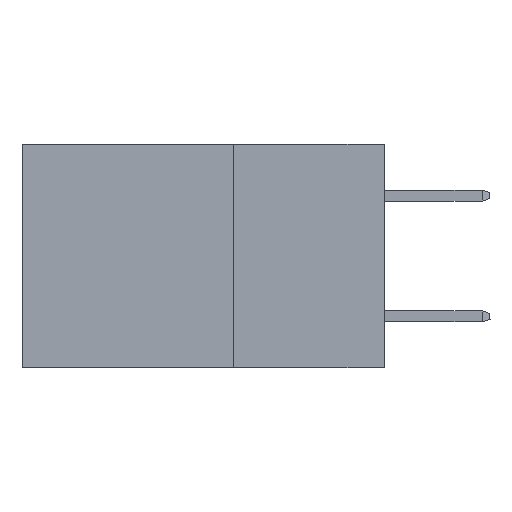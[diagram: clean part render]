
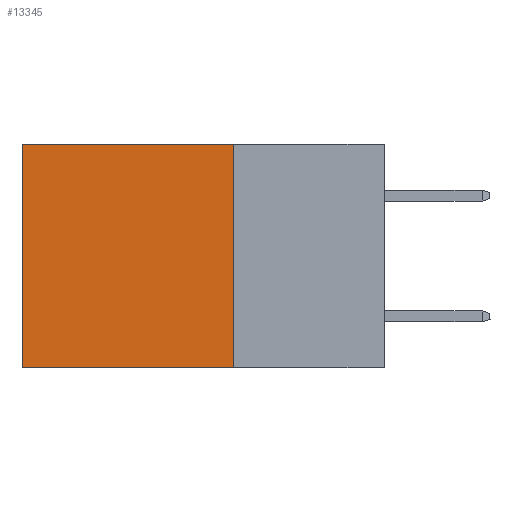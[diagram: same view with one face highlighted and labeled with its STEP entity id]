
A CAD part, left-side view. The second image highlights one B-rep face of the part: STEP entity #13345.
In plain terms, the highlighted planar face has unit normal (-1, 0, 0).
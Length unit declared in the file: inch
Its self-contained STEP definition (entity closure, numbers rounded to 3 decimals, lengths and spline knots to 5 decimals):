
#334 = FACE_OUTER_BOUND ( 'NONE', #6549, .T. ) ;
#1135 = AXIS2_PLACEMENT_3D ( 'NONE', #13825, #11307, #3402 ) ;
#1557 = CARTESIAN_POINT ( 'NONE',  ( 0.2615, 0.25, -0.37 ) ) ;
#1732 = ORIENTED_EDGE ( 'NONE', *, *, #14324, .F. ) ;
#2180 = EDGE_CURVE ( 'NONE', #16026, #10590, #16599, .T. ) ;
#2616 = CARTESIAN_POINT ( 'NONE',  ( 0.2615, 0.25, -0.37 ) ) ;
#2719 = VECTOR ( 'NONE', #7055, 39.37008 ) ;
#2734 = DIRECTION ( 'NONE',  ( 0., 1., 0. ) ) ;
#2771 = CARTESIAN_POINT ( 'NONE',  ( 0.2615, 0.25, 0. ) ) ;
#3402 = DIRECTION ( 'NONE',  ( 0., 0., -1. ) ) ;
#4527 = CARTESIAN_POINT ( 'NONE',  ( 0.2615, 0.6, -0.37 ) ) ;
#5103 = VECTOR ( 'NONE', #11102, 39.37008 ) ;
#5380 = EDGE_CURVE ( 'NONE', #10051, #6236, #15526, .T. ) ;
#5980 = PLANE ( 'NONE',  #1135 ) ;
#6153 = VECTOR ( 'NONE', #12124, 39.37008 ) ;
#6236 = VERTEX_POINT ( 'NONE', #4527 ) ;
#6471 = EDGE_CURVE ( 'NONE', #16026, #10051, #13386, .T. ) ;
#6549 = EDGE_LOOP ( 'NONE', ( #14987, #1732, #11427, #7682 ) ) ;
#7055 = DIRECTION ( 'NONE',  ( 0., 0., -1. ) ) ;
#7167 = CARTESIAN_POINT ( 'NONE',  ( 0.2615, 0.25, -0.37 ) ) ;
#7682 = ORIENTED_EDGE ( 'NONE', *, *, #6471, .T. ) ;
#9538 = CARTESIAN_POINT ( 'NONE',  ( 0.2615, 0.25, 0. ) ) ;
#10051 = VERTEX_POINT ( 'NONE', #16011 ) ;
#10590 = VERTEX_POINT ( 'NONE', #2616 ) ;
#11102 = DIRECTION ( 'NONE',  ( 0., 0., -1. ) ) ;
#11140 = CARTESIAN_POINT ( 'NONE',  ( 0.2615, 0.6, -0.37 ) ) ;
#11307 = DIRECTION ( 'NONE',  ( 1., 0., 0. ) ) ;
#11427 = ORIENTED_EDGE ( 'NONE', *, *, #2180, .F. ) ;
#12124 = DIRECTION ( 'NONE',  ( 0., 1., 0. ) ) ;
#13119 = LINE ( 'NONE', #1557, #6153 ) ;
#13345 = ADVANCED_FACE ( 'NONE', ( #334 ), #5980, .F. ) ;
#13386 = LINE ( 'NONE', #2771, #13794 ) ;
#13794 = VECTOR ( 'NONE', #2734, 39.37008 ) ;
#13825 = CARTESIAN_POINT ( 'NONE',  ( 0.2615, 0.25, -0.37 ) ) ;
#14324 = EDGE_CURVE ( 'NONE', #10590, #6236, #13119, .T. ) ;
#14987 = ORIENTED_EDGE ( 'NONE', *, *, #5380, .T. ) ;
#15526 = LINE ( 'NONE', #11140, #5103 ) ;
#16011 = CARTESIAN_POINT ( 'NONE',  ( 0.2615, 0.6, 0. ) ) ;
#16026 = VERTEX_POINT ( 'NONE', #9538 ) ;
#16599 = LINE ( 'NONE', #7167, #2719 ) ;
